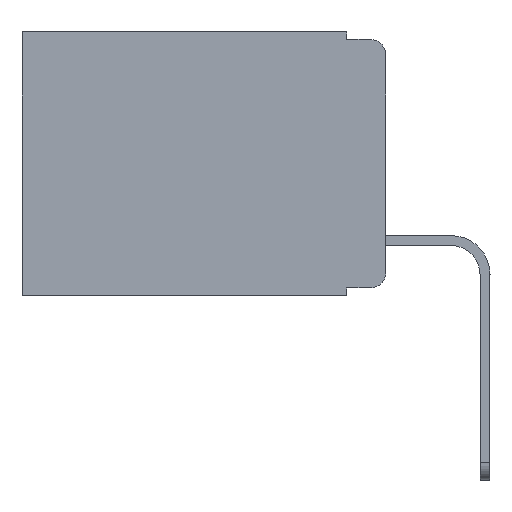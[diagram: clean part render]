
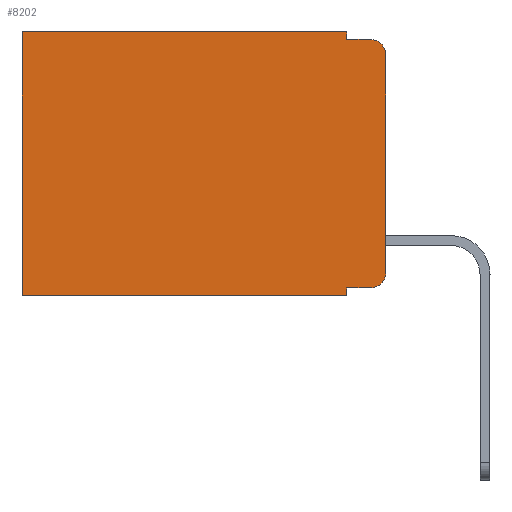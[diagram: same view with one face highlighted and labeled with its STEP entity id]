
A CAD part, left-side view. The second image highlights one B-rep face of the part: STEP entity #8202.
In plain terms, the highlighted planar face has unit normal (-1, 0, 0).
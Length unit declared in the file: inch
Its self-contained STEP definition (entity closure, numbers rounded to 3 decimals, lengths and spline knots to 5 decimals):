
#23 = LINE ( 'NONE', #7144, #5820 ) ;
#221 = LINE ( 'NONE', #224, #1362 ) ;
#224 = CARTESIAN_POINT ( 'NONE',  ( 0.298, 0.051, -0.01 ) ) ;
#249 = CARTESIAN_POINT ( 'NONE',  ( 0.298, 0.473, 0. ) ) ;
#274 = EDGE_CURVE ( 'NONE', #453, #7148, #10355, .T. ) ;
#336 = ORIENTED_EDGE ( 'NONE', *, *, #4727, .F. ) ;
#396 = DIRECTION ( 'NONE',  ( -1., 0., 0. ) ) ;
#423 = ORIENTED_EDGE ( 'NONE', *, *, #2972, .T. ) ;
#453 = VERTEX_POINT ( 'NONE', #11370 ) ;
#473 = CARTESIAN_POINT ( 'NONE',  ( 0.298, 0.02, -0.333 ) ) ;
#885 = CARTESIAN_POINT ( 'NONE',  ( 0.298, 0.02, -0.313 ) ) ;
#903 = EDGE_CURVE ( 'NONE', #2418, #8565, #1370, .T. ) ;
#1362 = VECTOR ( 'NONE', #3633, 39.37008 ) ;
#1370 = CIRCLE ( 'NONE', #5179, 0.02 ) ;
#1407 = DIRECTION ( 'NONE',  ( 0., 0., -1. ) ) ;
#1486 = DIRECTION ( 'NONE',  ( 0., 1., 0. ) ) ;
#1610 = VECTOR ( 'NONE', #5276, 39.37008 ) ;
#1708 = ORIENTED_EDGE ( 'NONE', *, *, #6597, .F. ) ;
#1728 = VECTOR ( 'NONE', #2581, 39.37008 ) ;
#1772 = ORIENTED_EDGE ( 'NONE', *, *, #903, .T. ) ;
#2296 = ORIENTED_EDGE ( 'NONE', *, *, #8987, .T. ) ;
#2418 = VERTEX_POINT ( 'NONE', #2856 ) ;
#2480 = CARTESIAN_POINT ( 'NONE',  ( 0.298, 0.051, 0. ) ) ;
#2581 = DIRECTION ( 'NONE',  ( 0., 0., -1. ) ) ;
#2856 = CARTESIAN_POINT ( 'NONE',  ( 0.298, 0., -0.03 ) ) ;
#2883 = LINE ( 'NONE', #7874, #5601 ) ;
#2972 = EDGE_CURVE ( 'NONE', #453, #8806, #8771, .T. ) ;
#3121 = DIRECTION ( 'NONE',  ( 0., 0., -1. ) ) ;
#3540 = DIRECTION ( 'NONE',  ( -1., 0., 0. ) ) ;
#3595 = EDGE_CURVE ( 'NONE', #2418, #7709, #5833, .T. ) ;
#3633 = DIRECTION ( 'NONE',  ( 0., -1., 0. ) ) ;
#3909 = CARTESIAN_POINT ( 'NONE',  ( 0.298, 0.051, 0. ) ) ;
#4131 = CIRCLE ( 'NONE', #8825, 0.02 ) ;
#4324 = DIRECTION ( 'NONE',  ( 0., 0., -1. ) ) ;
#4454 = CARTESIAN_POINT ( 'NONE',  ( 0.298, 0.473, -0.343 ) ) ;
#4636 = CARTESIAN_POINT ( 'NONE',  ( 0.298, 0.051, -0.01 ) ) ;
#4727 = EDGE_CURVE ( 'NONE', #4900, #9259, #8788, .T. ) ;
#4900 = VERTEX_POINT ( 'NONE', #2480 ) ;
#4950 = EDGE_CURVE ( 'NONE', #8806, #7709, #4131, .T. ) ;
#5179 = AXIS2_PLACEMENT_3D ( 'NONE', #7493, #396, #6706 ) ;
#5276 = DIRECTION ( 'NONE',  ( 0., -1., 0. ) ) ;
#5309 = CARTESIAN_POINT ( 'NONE',  ( 0.298, 0., -0.313 ) ) ;
#5601 = VECTOR ( 'NONE', #4324, 39.37008 ) ;
#5820 = VECTOR ( 'NONE', #6328, 39.37008 ) ;
#5833 = LINE ( 'NONE', #7034, #1728 ) ;
#5907 = PLANE ( 'NONE',  #10999 ) ;
#6152 = ORIENTED_EDGE ( 'NONE', *, *, #274, .F. ) ;
#6328 = DIRECTION ( 'NONE',  ( 0., 1., 0. ) ) ;
#6339 = FACE_OUTER_BOUND ( 'NONE', #8109, .T. ) ;
#6597 = EDGE_CURVE ( 'NONE', #7148, #6646, #23, .T. ) ;
#6646 = VERTEX_POINT ( 'NONE', #4454 ) ;
#6706 = DIRECTION ( 'NONE',  ( 0., 0., -1. ) ) ;
#6800 = DIRECTION ( 'NONE',  ( 1., 0., 0. ) ) ;
#7034 = CARTESIAN_POINT ( 'NONE',  ( 0.298, 0., 0. ) ) ;
#7144 = CARTESIAN_POINT ( 'NONE',  ( 0.298, 0., -0.343 ) ) ;
#7148 = VERTEX_POINT ( 'NONE', #7949 ) ;
#7333 = ORIENTED_EDGE ( 'NONE', *, *, #9263, .F. ) ;
#7392 = VECTOR ( 'NONE', #7696, 39.37008 ) ;
#7493 = CARTESIAN_POINT ( 'NONE',  ( 0.298, 0.02, -0.03 ) ) ;
#7582 = VECTOR ( 'NONE', #1486, 39.37008 ) ;
#7625 = CARTESIAN_POINT ( 'NONE',  ( 0.298, 0.051, 0. ) ) ;
#7696 = DIRECTION ( 'NONE',  ( 0., 0., -1. ) ) ;
#7709 = VERTEX_POINT ( 'NONE', #5309 ) ;
#7874 = CARTESIAN_POINT ( 'NONE',  ( 0.298, 0.473, 0. ) ) ;
#7949 = CARTESIAN_POINT ( 'NONE',  ( 0.298, 0.051, -0.343 ) ) ;
#7993 = VERTEX_POINT ( 'NONE', #249 ) ;
#8020 = ORIENTED_EDGE ( 'NONE', *, *, #4950, .T. ) ;
#8107 = ORIENTED_EDGE ( 'NONE', *, *, #3595, .F. ) ;
#8109 = EDGE_LOOP ( 'NONE', ( #8107, #1772, #7333, #336, #8350, #2296, #1708, #6152, #423, #8020 ) ) ;
#8202 = ADVANCED_FACE ( 'NONE', ( #6339 ), #5907, .F. ) ;
#8253 = VECTOR ( 'NONE', #3121, 39.37008 ) ;
#8332 = EDGE_CURVE ( 'NONE', #4900, #7993, #11202, .T. ) ;
#8350 = ORIENTED_EDGE ( 'NONE', *, *, #8332, .T. ) ;
#8565 = VERTEX_POINT ( 'NONE', #9011 ) ;
#8771 = LINE ( 'NONE', #10630, #1610 ) ;
#8788 = LINE ( 'NONE', #7625, #7392 ) ;
#8806 = VERTEX_POINT ( 'NONE', #473 ) ;
#8825 = AXIS2_PLACEMENT_3D ( 'NONE', #885, #3540, #9844 ) ;
#8987 = EDGE_CURVE ( 'NONE', #7993, #6646, #2883, .T. ) ;
#9011 = CARTESIAN_POINT ( 'NONE',  ( 0.298, 0.02, -0.01 ) ) ;
#9259 = VERTEX_POINT ( 'NONE', #4636 ) ;
#9263 = EDGE_CURVE ( 'NONE', #9259, #8565, #221, .T. ) ;
#9844 = DIRECTION ( 'NONE',  ( 0., 0., -1. ) ) ;
#10355 = LINE ( 'NONE', #3909, #8253 ) ;
#10630 = CARTESIAN_POINT ( 'NONE',  ( 0.298, 0.051, -0.333 ) ) ;
#10999 = AXIS2_PLACEMENT_3D ( 'NONE', #11080, #6800, #1407 ) ;
#11080 = CARTESIAN_POINT ( 'NONE',  ( 0.298, 0., 0. ) ) ;
#11202 = LINE ( 'NONE', #11426, #7582 ) ;
#11370 = CARTESIAN_POINT ( 'NONE',  ( 0.298, 0.051, -0.333 ) ) ;
#11426 = CARTESIAN_POINT ( 'NONE',  ( 0.298, 0., 0. ) ) ;
